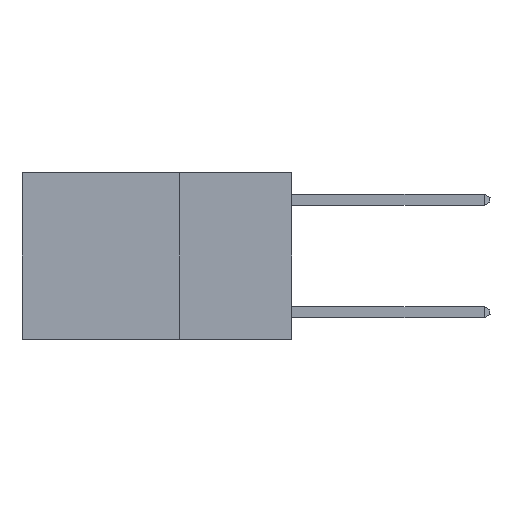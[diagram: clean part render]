
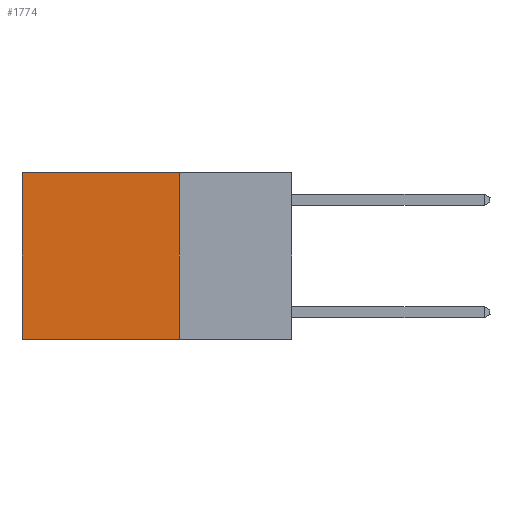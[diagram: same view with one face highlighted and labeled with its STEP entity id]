
A CAD part, left-side view. The second image highlights one B-rep face of the part: STEP entity #1774.
In plain terms, the highlighted planar face has unit normal (-1, 0, 0).
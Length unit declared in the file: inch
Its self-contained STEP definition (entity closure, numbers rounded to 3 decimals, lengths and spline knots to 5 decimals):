
#331 = DIRECTION ( 'NONE',  ( 0., 0., -1. ) ) ;
#548 = CARTESIAN_POINT ( 'NONE',  ( 0.2625, 0.25, 0. ) ) ;
#640 = VECTOR ( 'NONE', #4956, 39.37008 ) ;
#661 = VERTEX_POINT ( 'NONE', #10271 ) ;
#1106 = ORIENTED_EDGE ( 'NONE', *, *, #10219, .F. ) ;
#1250 = ORIENTED_EDGE ( 'NONE', *, *, #6973, .T. ) ;
#1393 = CARTESIAN_POINT ( 'NONE',  ( 0.2625, 0.25, -0.37 ) ) ;
#1532 = LINE ( 'NONE', #12505, #640 ) ;
#1774 = ADVANCED_FACE ( 'NONE', ( #5397 ), #9971, .F. ) ;
#2368 = CARTESIAN_POINT ( 'NONE',  ( 0.2625, 0.6, 0. ) ) ;
#2669 = ORIENTED_EDGE ( 'NONE', *, *, #11200, .F. ) ;
#2862 = CARTESIAN_POINT ( 'NONE',  ( 0.2625, 0.6, 0. ) ) ;
#3576 = ORIENTED_EDGE ( 'NONE', *, *, #11251, .T. ) ;
#4956 = DIRECTION ( 'NONE',  ( 0., 1., 0. ) ) ;
#5262 = DIRECTION ( 'NONE',  ( 1., 0., 0. ) ) ;
#5397 = FACE_OUTER_BOUND ( 'NONE', #10133, .T. ) ;
#6828 = VERTEX_POINT ( 'NONE', #13455 ) ;
#6973 = EDGE_CURVE ( 'NONE', #9283, #661, #14335, .T. ) ;
#7268 = LINE ( 'NONE', #11958, #14577 ) ;
#7595 = VECTOR ( 'NONE', #9527, 39.37008 ) ;
#9283 = VERTEX_POINT ( 'NONE', #2368 ) ;
#9527 = DIRECTION ( 'NONE',  ( 0., 1., 0. ) ) ;
#9971 = PLANE ( 'NONE',  #11220 ) ;
#10133 = EDGE_LOOP ( 'NONE', ( #1250, #2669, #1106, #3576 ) ) ;
#10219 = EDGE_CURVE ( 'NONE', #6828, #11481, #7268, .T. ) ;
#10271 = CARTESIAN_POINT ( 'NONE',  ( 0.2625, 0.6, -0.37 ) ) ;
#10776 = VECTOR ( 'NONE', #10916, 39.37008 ) ;
#10916 = DIRECTION ( 'NONE',  ( 0., 0., -1. ) ) ;
#11200 = EDGE_CURVE ( 'NONE', #11481, #661, #14857, .T. ) ;
#11220 = AXIS2_PLACEMENT_3D ( 'NONE', #548, #5262, #14602 ) ;
#11251 = EDGE_CURVE ( 'NONE', #6828, #9283, #1532, .T. ) ;
#11481 = VERTEX_POINT ( 'NONE', #12381 ) ;
#11958 = CARTESIAN_POINT ( 'NONE',  ( 0.2625, 0.25, 0. ) ) ;
#12381 = CARTESIAN_POINT ( 'NONE',  ( 0.2625, 0.25, -0.37 ) ) ;
#12505 = CARTESIAN_POINT ( 'NONE',  ( 0.2625, 0.25, 0. ) ) ;
#13455 = CARTESIAN_POINT ( 'NONE',  ( 0.2625, 0.25, 0. ) ) ;
#14335 = LINE ( 'NONE', #2862, #10776 ) ;
#14577 = VECTOR ( 'NONE', #331, 39.37008 ) ;
#14602 = DIRECTION ( 'NONE',  ( 0., 0., -1. ) ) ;
#14857 = LINE ( 'NONE', #1393, #7595 ) ;
